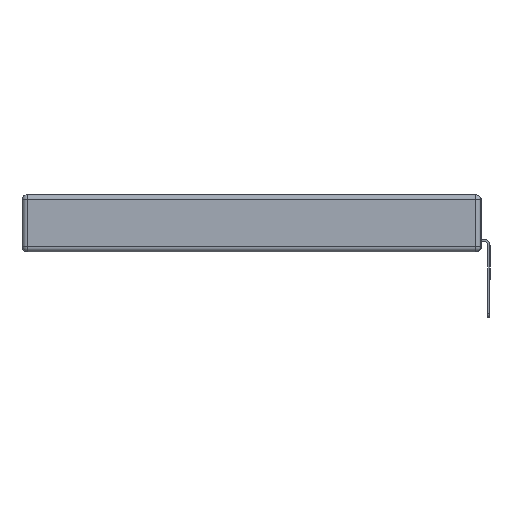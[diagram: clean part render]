
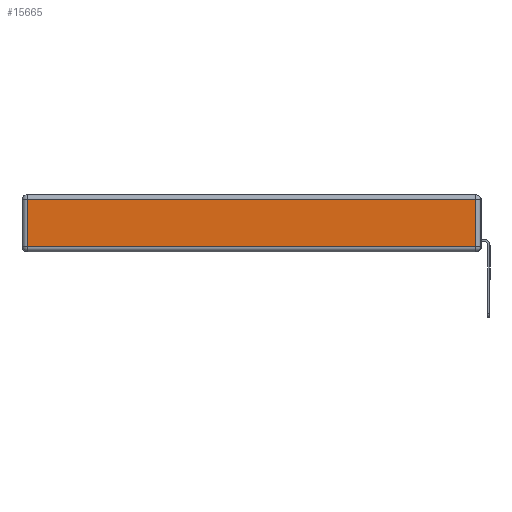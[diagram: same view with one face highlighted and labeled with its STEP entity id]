
A CAD part, left-side view. The second image highlights one B-rep face of the part: STEP entity #15665.
In plain terms, the highlighted planar face has unit normal (-1, 0, 0).
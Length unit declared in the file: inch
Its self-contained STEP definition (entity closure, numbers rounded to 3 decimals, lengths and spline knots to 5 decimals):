
#477 = ORIENTED_EDGE ( 'NONE', *, *, #5075, .T. ) ;
#1083 = AXIS2_PLACEMENT_3D ( 'NONE', #12918, #14448, #4034 ) ;
#1211 = CARTESIAN_POINT ( 'NONE',  ( 0., 2.72, -0.313 ) ) ;
#1694 = CARTESIAN_POINT ( 'NONE',  ( 0., 0.03, -0.03 ) ) ;
#2205 = VERTEX_POINT ( 'NONE', #1694 ) ;
#2509 = FACE_OUTER_BOUND ( 'NONE', #6396, .T. ) ;
#2767 = DIRECTION ( 'NONE',  ( 0., 0., -1. ) ) ;
#2924 = ORIENTED_EDGE ( 'NONE', *, *, #7602, .T. ) ;
#3301 = VERTEX_POINT ( 'NONE', #6065 ) ;
#4034 = DIRECTION ( 'NONE',  ( 0., 0., 1. ) ) ;
#4156 = ORIENTED_EDGE ( 'NONE', *, *, #15888, .T. ) ;
#4369 = CARTESIAN_POINT ( 'NONE',  ( 0., 2.75, -0.03 ) ) ;
#5018 = DIRECTION ( 'NONE',  ( 0., -1., 0. ) ) ;
#5075 = EDGE_CURVE ( 'NONE', #8954, #3301, #11519, .T. ) ;
#6042 = VERTEX_POINT ( 'NONE', #6347 ) ;
#6046 = ORIENTED_EDGE ( 'NONE', *, *, #9863, .T. ) ;
#6065 = CARTESIAN_POINT ( 'NONE',  ( 0., 0.03, -0.313 ) ) ;
#6347 = CARTESIAN_POINT ( 'NONE',  ( 0., 2.72, -0.03 ) ) ;
#6396 = EDGE_LOOP ( 'NONE', ( #477, #2924, #4156, #6046 ) ) ;
#6446 = CARTESIAN_POINT ( 'NONE',  ( 0., 2.72, -0.343 ) ) ;
#7183 = LINE ( 'NONE', #15214, #12697 ) ;
#7602 = EDGE_CURVE ( 'NONE', #3301, #2205, #7183, .T. ) ;
#7872 = VECTOR ( 'NONE', #5018, 39.37008 ) ;
#8954 = VERTEX_POINT ( 'NONE', #1211 ) ;
#9863 = EDGE_CURVE ( 'NONE', #6042, #8954, #14465, .T. ) ;
#9968 = VECTOR ( 'NONE', #2767, 39.37008 ) ;
#11519 = LINE ( 'NONE', #16718, #7872 ) ;
#11989 = VECTOR ( 'NONE', #14780, 39.37008 ) ;
#12397 = DIRECTION ( 'NONE',  ( 0., 0., 1. ) ) ;
#12697 = VECTOR ( 'NONE', #12397, 39.37008 ) ;
#12918 = CARTESIAN_POINT ( 'NONE',  ( 0., 0., -0.343 ) ) ;
#14123 = PLANE ( 'NONE',  #1083 ) ;
#14448 = DIRECTION ( 'NONE',  ( -1., 0., 0. ) ) ;
#14465 = LINE ( 'NONE', #6446, #9968 ) ;
#14780 = DIRECTION ( 'NONE',  ( 0., 1., 0. ) ) ;
#15214 = CARTESIAN_POINT ( 'NONE',  ( 0., 0.03, -0.343 ) ) ;
#15665 = ADVANCED_FACE ( 'NONE', ( #2509 ), #14123, .T. ) ;
#15888 = EDGE_CURVE ( 'NONE', #2205, #6042, #16065, .T. ) ;
#16065 = LINE ( 'NONE', #4369, #11989 ) ;
#16718 = CARTESIAN_POINT ( 'NONE',  ( 0., 0., -0.313 ) ) ;
